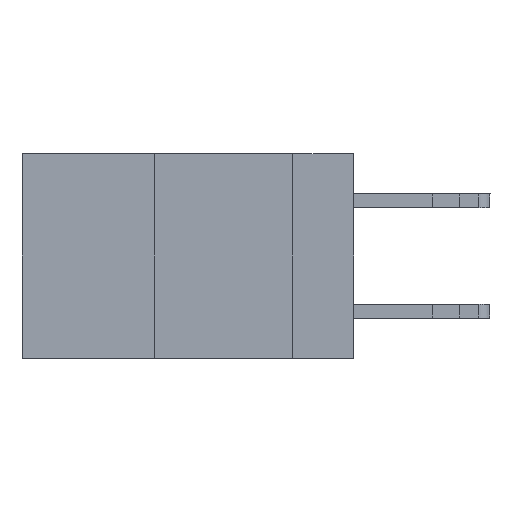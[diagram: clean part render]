
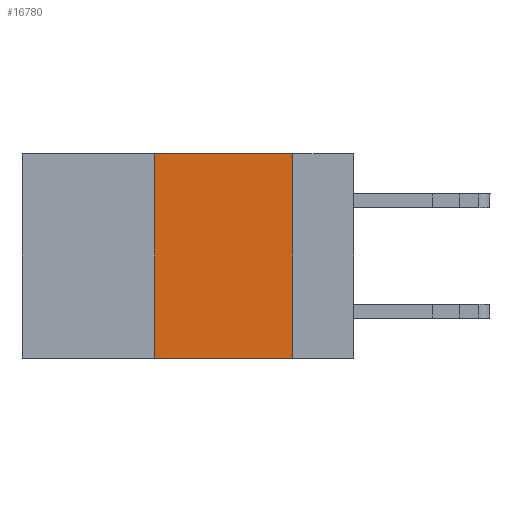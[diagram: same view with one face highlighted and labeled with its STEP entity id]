
A CAD part, left-side view. The second image highlights one B-rep face of the part: STEP entity #16780.
In plain terms, the highlighted planar face has unit normal (-1, 0, 0).
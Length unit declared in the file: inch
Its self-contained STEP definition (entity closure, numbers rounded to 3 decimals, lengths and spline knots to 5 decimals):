
#1401 = ORIENTED_EDGE ( 'NONE', *, *, #18223, .T. ) ;
#1524 = DIRECTION ( 'NONE',  ( 1., 0., 0. ) ) ;
#1735 = CARTESIAN_POINT ( 'NONE',  ( 0., 0.11, 0. ) ) ;
#2125 = CARTESIAN_POINT ( 'NONE',  ( 0., 0.36, -0.37 ) ) ;
#2514 = ORIENTED_EDGE ( 'NONE', *, *, #19577, .F. ) ;
#2886 = CARTESIAN_POINT ( 'NONE',  ( 0., 0.6, -0.37 ) ) ;
#3634 = VECTOR ( 'NONE', #14399, 39.37008 ) ;
#3801 = VERTEX_POINT ( 'NONE', #8876 ) ;
#4049 = VERTEX_POINT ( 'NONE', #15877 ) ;
#4502 = FACE_OUTER_BOUND ( 'NONE', #20079, .T. ) ;
#4588 = VERTEX_POINT ( 'NONE', #12407 ) ;
#4815 = CARTESIAN_POINT ( 'NONE',  ( 0., 0.6, 0. ) ) ;
#5058 = VECTOR ( 'NONE', #9183, 39.37008 ) ;
#7077 = VECTOR ( 'NONE', #10991, 39.37008 ) ;
#7502 = CARTESIAN_POINT ( 'NONE',  ( 0., 0.36, 0. ) ) ;
#8196 = PLANE ( 'NONE',  #15749 ) ;
#8876 = CARTESIAN_POINT ( 'NONE',  ( 0., 0.11, -0.37 ) ) ;
#9183 = DIRECTION ( 'NONE',  ( 0., 0., 1. ) ) ;
#9493 = LINE ( 'NONE', #7502, #5058 ) ;
#10859 = ORIENTED_EDGE ( 'NONE', *, *, #11854, .F. ) ;
#10991 = DIRECTION ( 'NONE',  ( 0., -1., 0. ) ) ;
#11854 = EDGE_CURVE ( 'NONE', #21331, #4588, #9493, .T. ) ;
#12407 = CARTESIAN_POINT ( 'NONE',  ( 0., 0.36, 0. ) ) ;
#12482 = LINE ( 'NONE', #1735, #16768 ) ;
#13105 = DIRECTION ( 'NONE',  ( 0., 0., -1. ) ) ;
#13302 = DIRECTION ( 'NONE',  ( 0., 0., -1. ) ) ;
#13926 = ORIENTED_EDGE ( 'NONE', *, *, #17485, .F. ) ;
#14399 = DIRECTION ( 'NONE',  ( 0., -1., 0. ) ) ;
#15749 = AXIS2_PLACEMENT_3D ( 'NONE', #4815, #1524, #13105 ) ;
#15877 = CARTESIAN_POINT ( 'NONE',  ( 0., 0.11, 0. ) ) ;
#16768 = VECTOR ( 'NONE', #13302, 39.37008 ) ;
#16780 = ADVANCED_FACE ( 'NONE', ( #4502 ), #8196, .F. ) ;
#17485 = EDGE_CURVE ( 'NONE', #4588, #4049, #20094, .T. ) ;
#18223 = EDGE_CURVE ( 'NONE', #21331, #3801, #21064, .T. ) ;
#19577 = EDGE_CURVE ( 'NONE', #4049, #3801, #12482, .T. ) ;
#20079 = EDGE_LOOP ( 'NONE', ( #2514, #13926, #10859, #1401 ) ) ;
#20094 = LINE ( 'NONE', #20684, #7077 ) ;
#20684 = CARTESIAN_POINT ( 'NONE',  ( 0., 0.6, 0. ) ) ;
#21064 = LINE ( 'NONE', #2886, #3634 ) ;
#21331 = VERTEX_POINT ( 'NONE', #2125 ) ;
